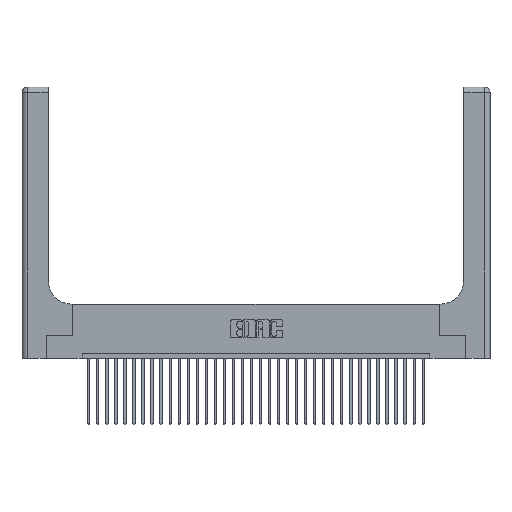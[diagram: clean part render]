
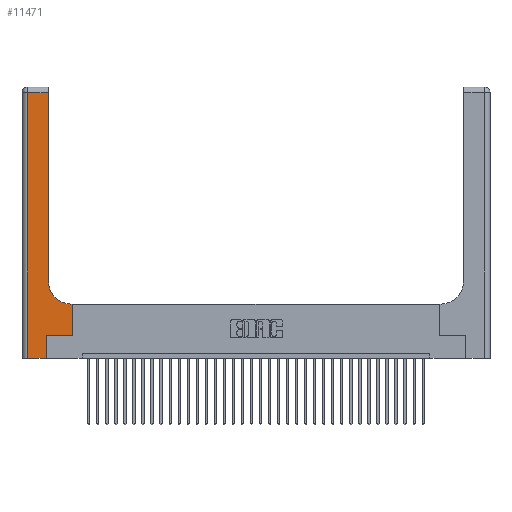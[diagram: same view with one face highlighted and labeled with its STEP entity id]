
A CAD part, top view. The second image highlights one B-rep face of the part: STEP entity #11471.
In plain terms, the highlighted planar face has unit normal (0, 0, 1).
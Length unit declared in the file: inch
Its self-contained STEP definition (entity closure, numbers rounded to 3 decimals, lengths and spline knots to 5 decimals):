
#135 = ORIENTED_EDGE ( 'NONE', *, *, #7928, .T. ) ;
#500 = CARTESIAN_POINT ( 'NONE',  ( 0.269, 0.25, 0.37 ) ) ;
#636 = DIRECTION ( 'NONE',  ( 0., 1., 0. ) ) ;
#741 = CARTESIAN_POINT ( 'NONE',  ( 0.269, 0., 0.37 ) ) ;
#805 = CARTESIAN_POINT ( 'NONE',  ( 0.2915, 2.94, 0.37 ) ) ;
#894 = DIRECTION ( 'NONE',  ( 0., 0., -1. ) ) ;
#1480 = VERTEX_POINT ( 'NONE', #18433 ) ;
#2126 = VECTOR ( 'NONE', #27076, 39.37008 ) ;
#2606 = CARTESIAN_POINT ( 'NONE',  ( 0.2915, 3., 0.37 ) ) ;
#2702 = ORIENTED_EDGE ( 'NONE', *, *, #9296, .T. ) ;
#2751 = VECTOR ( 'NONE', #5516, 39.37008 ) ;
#3375 = ORIENTED_EDGE ( 'NONE', *, *, #22694, .T. ) ;
#3479 = LINE ( 'NONE', #2606, #15940 ) ;
#3965 = ORIENTED_EDGE ( 'NONE', *, *, #9030, .T. ) ;
#4953 = DIRECTION ( 'NONE',  ( 0., 1., 0. ) ) ;
#5516 = DIRECTION ( 'NONE',  ( 1., 0., 0. ) ) ;
#5858 = LINE ( 'NONE', #32691, #24140 ) ;
#6106 = DIRECTION ( 'NONE',  ( -1., 0., 0. ) ) ;
#6107 = DIRECTION ( 'NONE',  ( -1., 0., 0. ) ) ;
#6594 = LINE ( 'NONE', #741, #13238 ) ;
#6616 = VERTEX_POINT ( 'NONE', #805 ) ;
#6892 = LINE ( 'NONE', #18058, #13117 ) ;
#6932 = CARTESIAN_POINT ( 'NONE',  ( 0.06, 2.94, 0.37 ) ) ;
#7789 = FACE_OUTER_BOUND ( 'NONE', #25271, .T. ) ;
#7811 = ORIENTED_EDGE ( 'NONE', *, *, #32948, .T. ) ;
#7928 = EDGE_CURVE ( 'NONE', #30454, #23058, #33268, .T. ) ;
#8050 = DIRECTION ( 'NONE',  ( 0., 1., 0. ) ) ;
#8146 = LINE ( 'NONE', #23980, #2751 ) ;
#9030 = EDGE_CURVE ( 'NONE', #33339, #30454, #5858, .T. ) ;
#9296 = EDGE_CURVE ( 'NONE', #6616, #32504, #29489, .T. ) ;
#10867 = VECTOR ( 'NONE', #6106, 39.37008 ) ;
#11471 = ADVANCED_FACE ( 'NONE', ( #7789 ), #17393, .F. ) ;
#12212 = DIRECTION ( 'NONE',  ( 0., -1., 0. ) ) ;
#12237 = LINE ( 'NONE', #14280, #32083 ) ;
#12937 = VERTEX_POINT ( 'NONE', #24251 ) ;
#13117 = VECTOR ( 'NONE', #4953, 39.37008 ) ;
#13207 = EDGE_CURVE ( 'NONE', #32504, #30427, #12237, .T. ) ;
#13238 = VECTOR ( 'NONE', #636, 39.37008 ) ;
#14280 = CARTESIAN_POINT ( 'NONE',  ( 0.06, 3., 0.37 ) ) ;
#15940 = VECTOR ( 'NONE', #8050, 39.37008 ) ;
#16888 = AXIS2_PLACEMENT_3D ( 'NONE', #19803, #894, #27461 ) ;
#17393 = PLANE ( 'NONE',  #18757 ) ;
#17617 = EDGE_CURVE ( 'NONE', #30427, #1480, #8146, .T. ) ;
#18058 = CARTESIAN_POINT ( 'NONE',  ( 0.5585, 0.25, 0.37 ) ) ;
#18433 = CARTESIAN_POINT ( 'NONE',  ( 0.269, 0., 0.37 ) ) ;
#18757 = AXIS2_PLACEMENT_3D ( 'NONE', #33386, #30834, #6107 ) ;
#19803 = CARTESIAN_POINT ( 'NONE',  ( 0.5415, 0.85, 0.37 ) ) ;
#19991 = VERTEX_POINT ( 'NONE', #30452 ) ;
#20816 = CARTESIAN_POINT ( 'NONE',  ( 0.5585, 0.6, 0.37 ) ) ;
#21650 = EDGE_CURVE ( 'NONE', #19991, #33339, #6892, .T. ) ;
#22186 = DIRECTION ( 'NONE',  ( -1., 0., 0. ) ) ;
#22694 = EDGE_CURVE ( 'NONE', #23058, #6616, #3479, .T. ) ;
#23058 = VERTEX_POINT ( 'NONE', #34065 ) ;
#23980 = CARTESIAN_POINT ( 'NONE',  ( 0., 0., 0.37 ) ) ;
#24140 = VECTOR ( 'NONE', #22186, 39.37008 ) ;
#24251 = CARTESIAN_POINT ( 'NONE',  ( 0.269, 0.25, 0.37 ) ) ;
#25271 = EDGE_LOOP ( 'NONE', ( #3375, #2702, #26918, #32197, #32940, #7811, #31487, #3965, #135 ) ) ;
#25781 = LINE ( 'NONE', #500, #2126 ) ;
#25902 = EDGE_CURVE ( 'NONE', #1480, #12937, #6594, .T. ) ;
#25968 = CARTESIAN_POINT ( 'NONE',  ( 0.5415, 0.6, 0.37 ) ) ;
#26918 = ORIENTED_EDGE ( 'NONE', *, *, #13207, .T. ) ;
#27076 = DIRECTION ( 'NONE',  ( 1., 0., 0. ) ) ;
#27461 = DIRECTION ( 'NONE',  ( 1., 0., 0. ) ) ;
#27465 = CARTESIAN_POINT ( 'NONE',  ( 0., 2.94, 0.37 ) ) ;
#29489 = LINE ( 'NONE', #27465, #10867 ) ;
#30427 = VERTEX_POINT ( 'NONE', #34059 ) ;
#30452 = CARTESIAN_POINT ( 'NONE',  ( 0.5585, 0.25, 0.37 ) ) ;
#30454 = VERTEX_POINT ( 'NONE', #25968 ) ;
#30834 = DIRECTION ( 'NONE',  ( 0., 0., -1. ) ) ;
#31487 = ORIENTED_EDGE ( 'NONE', *, *, #21650, .T. ) ;
#32083 = VECTOR ( 'NONE', #12212, 39.37008 ) ;
#32197 = ORIENTED_EDGE ( 'NONE', *, *, #17617, .T. ) ;
#32504 = VERTEX_POINT ( 'NONE', #6932 ) ;
#32691 = CARTESIAN_POINT ( 'NONE',  ( 0.2915, 0.6, 0.37 ) ) ;
#32940 = ORIENTED_EDGE ( 'NONE', *, *, #25902, .T. ) ;
#32948 = EDGE_CURVE ( 'NONE', #12937, #19991, #25781, .T. ) ;
#33268 = CIRCLE ( 'NONE', #16888, 0.25 ) ;
#33339 = VERTEX_POINT ( 'NONE', #20816 ) ;
#33386 = CARTESIAN_POINT ( 'NONE',  ( 0., 3., 0.37 ) ) ;
#34059 = CARTESIAN_POINT ( 'NONE',  ( 0.06, 0., 0.37 ) ) ;
#34065 = CARTESIAN_POINT ( 'NONE',  ( 0.2915, 0.85, 0.37 ) ) ;
